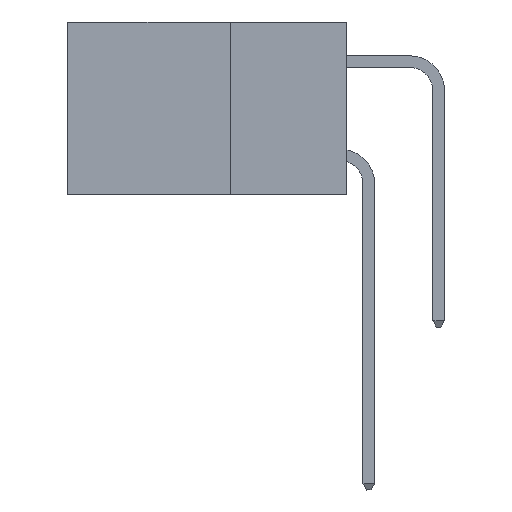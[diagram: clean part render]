
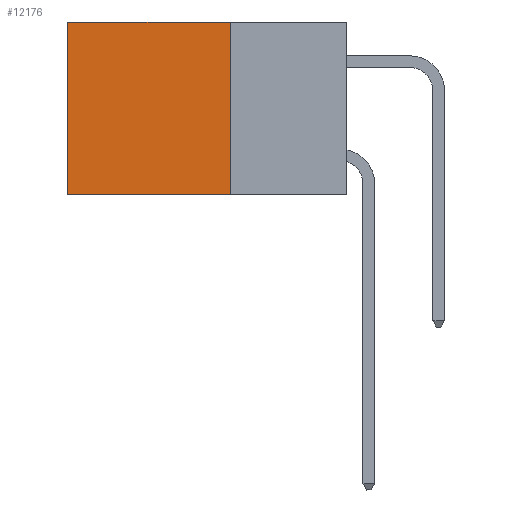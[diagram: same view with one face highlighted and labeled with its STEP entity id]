
A CAD part, left-side view. The second image highlights one B-rep face of the part: STEP entity #12176.
In plain terms, the highlighted planar face has unit normal (-1, 0, 0).
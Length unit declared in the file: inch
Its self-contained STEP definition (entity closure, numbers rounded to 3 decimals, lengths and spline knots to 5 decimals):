
#2590 = DIRECTION ( 'NONE',  ( 0., 1., 0. ) ) ;
#3551 = EDGE_CURVE ( 'NONE', #15479, #13953, #5112, .T. ) ;
#4142 = VECTOR ( 'NONE', #15450, 39.37008 ) ;
#5112 = LINE ( 'NONE', #21881, #4142 ) ;
#5686 = VERTEX_POINT ( 'NONE', #27223 ) ;
#6381 = ORIENTED_EDGE ( 'NONE', *, *, #18625, .T. ) ;
#6708 = ORIENTED_EDGE ( 'NONE', *, *, #3551, .F. ) ;
#6816 = CARTESIAN_POINT ( 'NONE',  ( 0.2875, 0.25, 0. ) ) ;
#7314 = CARTESIAN_POINT ( 'NONE',  ( 0.2875, 0.25, 0. ) ) ;
#8167 = LINE ( 'NONE', #33241, #42412 ) ;
#8425 = ORIENTED_EDGE ( 'NONE', *, *, #18212, .T. ) ;
#10754 = PLANE ( 'NONE',  #14751 ) ;
#12176 = ADVANCED_FACE ( 'NONE', ( #13779 ), #10754, .F. ) ;
#12281 = CARTESIAN_POINT ( 'NONE',  ( 0.2875, 0.25, -0.37 ) ) ;
#13779 = FACE_OUTER_BOUND ( 'NONE', #14646, .T. ) ;
#13953 = VERTEX_POINT ( 'NONE', #12281 ) ;
#14646 = EDGE_LOOP ( 'NONE', ( #8425, #27733, #6708, #6381 ) ) ;
#14751 = AXIS2_PLACEMENT_3D ( 'NONE', #7314, #20453, #27808 ) ;
#15450 = DIRECTION ( 'NONE',  ( 0., 0., -1. ) ) ;
#15479 = VERTEX_POINT ( 'NONE', #6816 ) ;
#15786 = CARTESIAN_POINT ( 'NONE',  ( 0.2875, 0.6, 0. ) ) ;
#16412 = LINE ( 'NONE', #44711, #27635 ) ;
#17654 = VERTEX_POINT ( 'NONE', #22054 ) ;
#18212 = EDGE_CURVE ( 'NONE', #17654, #5686, #36524, .T. ) ;
#18625 = EDGE_CURVE ( 'NONE', #15479, #17654, #8167, .T. ) ;
#19254 = DIRECTION ( 'NONE',  ( 0., 0., -1. ) ) ;
#20453 = DIRECTION ( 'NONE',  ( 1., 0., 0. ) ) ;
#21881 = CARTESIAN_POINT ( 'NONE',  ( 0.2875, 0.25, 0. ) ) ;
#21945 = DIRECTION ( 'NONE',  ( 0., 1., 0. ) ) ;
#22054 = CARTESIAN_POINT ( 'NONE',  ( 0.2875, 0.6, 0. ) ) ;
#27223 = CARTESIAN_POINT ( 'NONE',  ( 0.2875, 0.6, -0.37 ) ) ;
#27635 = VECTOR ( 'NONE', #2590, 39.37008 ) ;
#27733 = ORIENTED_EDGE ( 'NONE', *, *, #41377, .F. ) ;
#27808 = DIRECTION ( 'NONE',  ( 0., 0., -1. ) ) ;
#33241 = CARTESIAN_POINT ( 'NONE',  ( 0.2875, 0.25, 0. ) ) ;
#36524 = LINE ( 'NONE', #15786, #38040 ) ;
#38040 = VECTOR ( 'NONE', #19254, 39.37008 ) ;
#41377 = EDGE_CURVE ( 'NONE', #13953, #5686, #16412, .T. ) ;
#42412 = VECTOR ( 'NONE', #21945, 39.37008 ) ;
#44711 = CARTESIAN_POINT ( 'NONE',  ( 0.2875, 0.25, -0.37 ) ) ;
